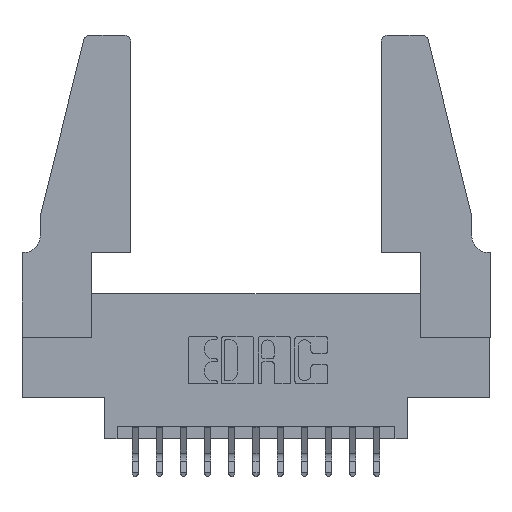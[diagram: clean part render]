
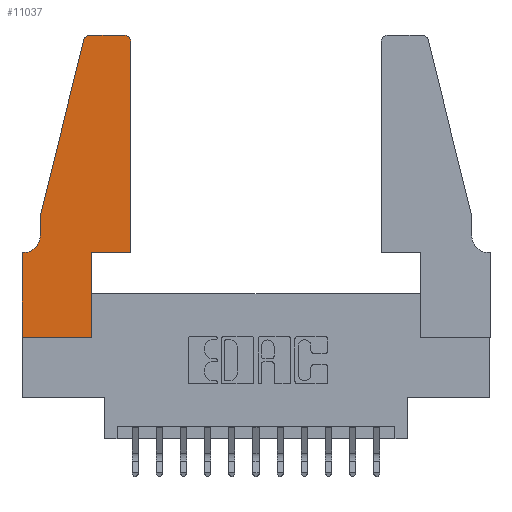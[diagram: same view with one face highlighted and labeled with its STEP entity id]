
A CAD part, top view. The second image highlights one B-rep face of the part: STEP entity #11037.
In plain terms, the highlighted planar face has unit normal (0, 0, 1).
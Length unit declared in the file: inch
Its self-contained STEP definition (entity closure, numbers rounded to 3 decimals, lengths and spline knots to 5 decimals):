
#33 = LINE ( 'NONE', #12486, #4858 ) ;
#211 = VERTEX_POINT ( 'NONE', #14274 ) ;
#451 = VERTEX_POINT ( 'NONE', #2880 ) ;
#552 = VERTEX_POINT ( 'NONE', #12438 ) ;
#677 = EDGE_CURVE ( 'NONE', #4146, #11160, #5043, .T. ) ;
#786 = ORIENTED_EDGE ( 'NONE', *, *, #11417, .T. ) ;
#957 = DIRECTION ( 'NONE',  ( -1., 0., 0. ) ) ;
#1021 = CARTESIAN_POINT ( 'NONE',  ( 0.2865, 0.35, 0.37 ) ) ;
#1110 = LINE ( 'NONE', #9858, #15159 ) ;
#1126 = CARTESIAN_POINT ( 'NONE',  ( 0.4205, 1.22, 0.37 ) ) ;
#1171 = CARTESIAN_POINT ( 'NONE',  ( 0.284, 1.22, 0.37 ) ) ;
#1429 = VERTEX_POINT ( 'NONE', #6427 ) ;
#1461 = EDGE_CURVE ( 'NONE', #5876, #10034, #14305, .T. ) ;
#1480 = CARTESIAN_POINT ( 'NONE',  ( 0.0755, 0.35, 0.37 ) ) ;
#1514 = EDGE_CURVE ( 'NONE', #11677, #4146, #3187, .T. ) ;
#1688 = VERTEX_POINT ( 'NONE', #2156 ) ;
#1844 = DIRECTION ( 'NONE',  ( -1., 0., 0. ) ) ;
#1962 = EDGE_CURVE ( 'NONE', #451, #6208, #4672, .T. ) ;
#2043 = CARTESIAN_POINT ( 'NONE',  ( 0.4505, 0.35, 0.37 ) ) ;
#2156 = CARTESIAN_POINT ( 'NONE',  ( 0.2865, 0.35, 0.37 ) ) ;
#2173 = CARTESIAN_POINT ( 'NONE',  ( 0.25487, 1.22718, 0.37 ) ) ;
#2559 = DIRECTION ( 'NONE',  ( -1., 0., 0. ) ) ;
#2672 = DIRECTION ( 'NONE',  ( 0., -1., 0. ) ) ;
#2820 = CARTESIAN_POINT ( 'NONE',  ( 0., 0., 0.37 ) ) ;
#2880 = CARTESIAN_POINT ( 'NONE',  ( 0.0755, 0.42, 0.37 ) ) ;
#3187 = LINE ( 'NONE', #6667, #9861 ) ;
#3401 = ORIENTED_EDGE ( 'NONE', *, *, #8201, .T. ) ;
#3457 = AXIS2_PLACEMENT_3D ( 'NONE', #6775, #5651, #6674 ) ;
#3626 = EDGE_CURVE ( 'NONE', #552, #12993, #5177, .T. ) ;
#3847 = CIRCLE ( 'NONE', #13383, 0.03 ) ;
#3907 = AXIS2_PLACEMENT_3D ( 'NONE', #1126, #12931, #8104 ) ;
#3914 = CARTESIAN_POINT ( 'NONE',  ( 0., 0., 0.37 ) ) ;
#4021 = EDGE_LOOP ( 'NONE', ( #10784, #9180, #8367, #786, #14602, #3401, #12566, #7311, #4562, #5273, #4795, #7577 ) ) ;
#4146 = VERTEX_POINT ( 'NONE', #9649 ) ;
#4562 = ORIENTED_EDGE ( 'NONE', *, *, #9870, .T. ) ;
#4672 = CIRCLE ( 'NONE', #11148, 0.07 ) ;
#4679 = DIRECTION ( 'NONE',  ( 1., 0., 0. ) ) ;
#4795 = ORIENTED_EDGE ( 'NONE', *, *, #1514, .T. ) ;
#4858 = VECTOR ( 'NONE', #1844, 39.37008 ) ;
#5043 = CIRCLE ( 'NONE', #3907, 0.03 ) ;
#5177 = LINE ( 'NONE', #3914, #13491 ) ;
#5273 = ORIENTED_EDGE ( 'NONE', *, *, #12742, .T. ) ;
#5651 = DIRECTION ( 'NONE',  ( 0., 0., 1. ) ) ;
#5876 = VERTEX_POINT ( 'NONE', #2173 ) ;
#5898 = EDGE_CURVE ( 'NONE', #12993, #211, #13996, .T. ) ;
#5947 = FACE_OUTER_BOUND ( 'NONE', #4021, .T. ) ;
#6208 = VERTEX_POINT ( 'NONE', #14178 ) ;
#6427 = CARTESIAN_POINT ( 'NONE',  ( 0.284, 1.25, 0.37 ) ) ;
#6667 = CARTESIAN_POINT ( 'NONE',  ( 0.4505, 0.35, 0.37 ) ) ;
#6674 = DIRECTION ( 'NONE',  ( 1., 0., 0. ) ) ;
#6703 = CARTESIAN_POINT ( 'NONE',  ( 0.4505, 0.35, 0.37 ) ) ;
#6775 = CARTESIAN_POINT ( 'NONE',  ( 0., 0.35, 0.37 ) ) ;
#7020 = DIRECTION ( 'NONE',  ( 0., 0., 1. ) ) ;
#7070 = CARTESIAN_POINT ( 'NONE',  ( 0.0755, 0.5, 0.37 ) ) ;
#7311 = ORIENTED_EDGE ( 'NONE', *, *, #5898, .T. ) ;
#7505 = DIRECTION ( 'NONE',  ( 0., -1., 0. ) ) ;
#7577 = ORIENTED_EDGE ( 'NONE', *, *, #677, .T. ) ;
#7861 = LINE ( 'NONE', #1480, #9524 ) ;
#7902 = VECTOR ( 'NONE', #11618, 39.37008 ) ;
#8104 = DIRECTION ( 'NONE',  ( 1., 0., 0. ) ) ;
#8201 = EDGE_CURVE ( 'NONE', #6208, #552, #7861, .T. ) ;
#8367 = ORIENTED_EDGE ( 'NONE', *, *, #1461, .T. ) ;
#8915 = LINE ( 'NONE', #1021, #10396 ) ;
#9048 = EDGE_CURVE ( 'NONE', #11160, #1429, #33, .T. ) ;
#9180 = ORIENTED_EDGE ( 'NONE', *, *, #11816, .T. ) ;
#9524 = VECTOR ( 'NONE', #957, 39.37008 ) ;
#9649 = CARTESIAN_POINT ( 'NONE',  ( 0.4505, 1.22, 0.37 ) ) ;
#9858 = CARTESIAN_POINT ( 'NONE',  ( 0.0755, 0.5, 0.37 ) ) ;
#9861 = VECTOR ( 'NONE', #13527, 39.37008 ) ;
#9870 = EDGE_CURVE ( 'NONE', #211, #1688, #8915, .T. ) ;
#10034 = VERTEX_POINT ( 'NONE', #7070 ) ;
#10187 = CARTESIAN_POINT ( 'NONE',  ( 0., 0., 0.37 ) ) ;
#10355 = DIRECTION ( 'NONE',  ( 0., 1., 0. ) ) ;
#10396 = VECTOR ( 'NONE', #10355, 39.37008 ) ;
#10784 = ORIENTED_EDGE ( 'NONE', *, *, #9048, .T. ) ;
#11037 = ADVANCED_FACE ( 'NONE', ( #5947 ), #12605, .T. ) ;
#11148 = AXIS2_PLACEMENT_3D ( 'NONE', #14505, #13264, #2559 ) ;
#11160 = VERTEX_POINT ( 'NONE', #14980 ) ;
#11207 = VECTOR ( 'NONE', #11620, 39.37008 ) ;
#11417 = EDGE_CURVE ( 'NONE', #10034, #451, #1110, .T. ) ;
#11618 = DIRECTION ( 'NONE',  ( 1., 0., 0. ) ) ;
#11620 = DIRECTION ( 'NONE',  ( 1., 0., 0. ) ) ;
#11677 = VERTEX_POINT ( 'NONE', #6703 ) ;
#11816 = EDGE_CURVE ( 'NONE', #1429, #5876, #3847, .T. ) ;
#12438 = CARTESIAN_POINT ( 'NONE',  ( 0., 0.35, 0.37 ) ) ;
#12486 = CARTESIAN_POINT ( 'NONE',  ( 0.2605, 1.25, 0.37 ) ) ;
#12566 = ORIENTED_EDGE ( 'NONE', *, *, #3626, .T. ) ;
#12605 = PLANE ( 'NONE',  #3457 ) ;
#12742 = EDGE_CURVE ( 'NONE', #1688, #11677, #12875, .T. ) ;
#12875 = LINE ( 'NONE', #2043, #7902 ) ;
#12931 = DIRECTION ( 'NONE',  ( 0., 0., 1. ) ) ;
#12993 = VERTEX_POINT ( 'NONE', #2820 ) ;
#13264 = DIRECTION ( 'NONE',  ( 0., 0., -1. ) ) ;
#13284 = CARTESIAN_POINT ( 'NONE',  ( 0.0755, 0.5, 0.37 ) ) ;
#13383 = AXIS2_PLACEMENT_3D ( 'NONE', #1171, #7020, #4679 ) ;
#13491 = VECTOR ( 'NONE', #7505, 39.37008 ) ;
#13527 = DIRECTION ( 'NONE',  ( 0., 1., 0. ) ) ;
#13996 = LINE ( 'NONE', #10187, #11207 ) ;
#14129 = VECTOR ( 'NONE', #14522, 39.37008 ) ;
#14178 = CARTESIAN_POINT ( 'NONE',  ( 0.0055, 0.35, 0.37 ) ) ;
#14274 = CARTESIAN_POINT ( 'NONE',  ( 0.2865, 0., 0.37 ) ) ;
#14305 = LINE ( 'NONE', #13284, #14129 ) ;
#14505 = CARTESIAN_POINT ( 'NONE',  ( 0.0055, 0.42, 0.37 ) ) ;
#14522 = DIRECTION ( 'NONE',  ( -0.239, -0.971, 0. ) ) ;
#14602 = ORIENTED_EDGE ( 'NONE', *, *, #1962, .T. ) ;
#14980 = CARTESIAN_POINT ( 'NONE',  ( 0.4205, 1.25, 0.37 ) ) ;
#15159 = VECTOR ( 'NONE', #2672, 39.37008 ) ;
